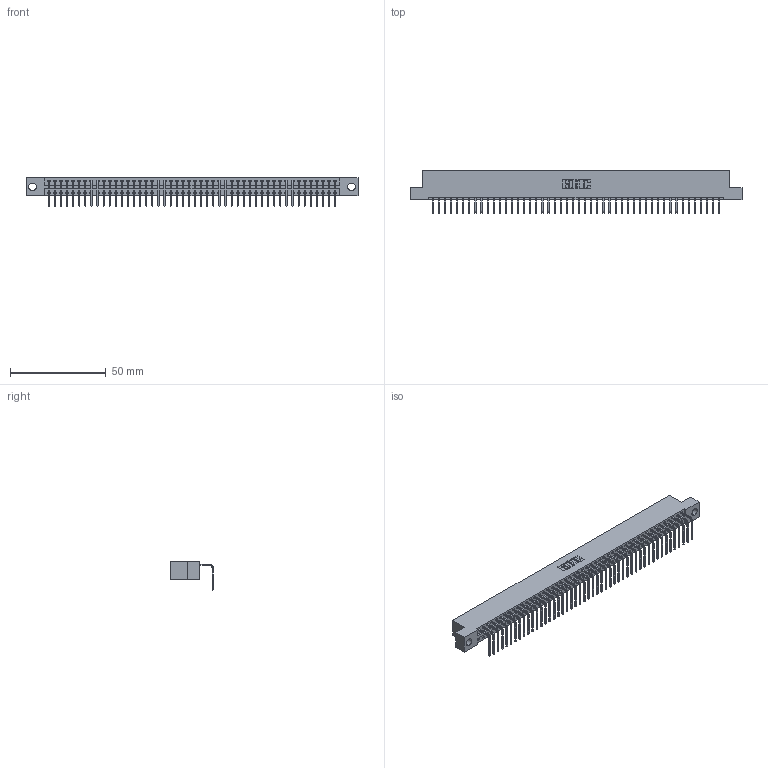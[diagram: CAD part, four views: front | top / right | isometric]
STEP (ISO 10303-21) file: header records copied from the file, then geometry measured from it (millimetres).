
FILE_DESCRIPTION (( 'STEP AP203' ), '1' );
FILE_NAME ('346-048-558-104.STEP', '2022-05-10T00:07:07', ( '' ), ( '' ), 'SwSTEP 2.0', 'SolidWorks 2020', '' );
FILE_SCHEMA (( 'CONFIG_CONTROL_DESIGN' ));
Length unit declared in the file: inch
Products named in the file (3): 345-292-001_558 Tail - 2; 346-048-558-104; 346 Part_Flush Mounting Lugs - 0.156 Dia-TH
Assembly tree (49 placements, depth 2):
  346-048-558-104
    346 Part_Flush Mounting Lugs - 0.156 Dia-TH
    345-292-001_558 Tail - 2  x48
Bounding box: 172.97 x 22.16 x 14.73 mm (x, y, z)
Volume: 16652.8 mm3; surface area: 21669.9 mm2
Topology: 49 solids, 49 shells, 3016 faces, 9101 edges, 6002 vertices
Faces by surface type: plane 2106, cylinder 910
Entity records: 29485 total; most frequent: CARTESIAN_POINT 5062, ORIENTED_EDGE 5042, DIRECTION 4457, EDGE_CURVE 2521, VECTOR 2197, LINE 2197, VERTEX_POINT 1678, AXIS2_PLACEMENT_3D 1130
